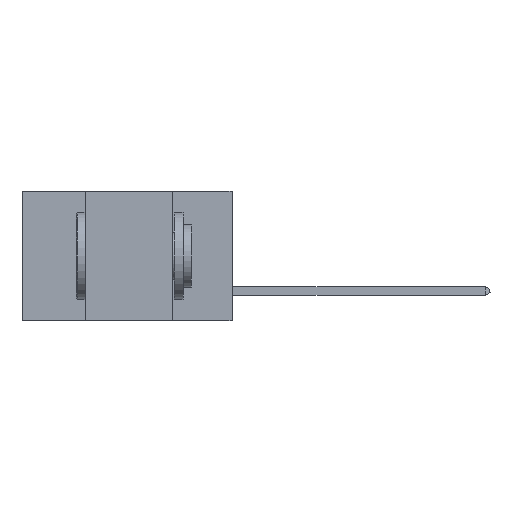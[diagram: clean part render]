
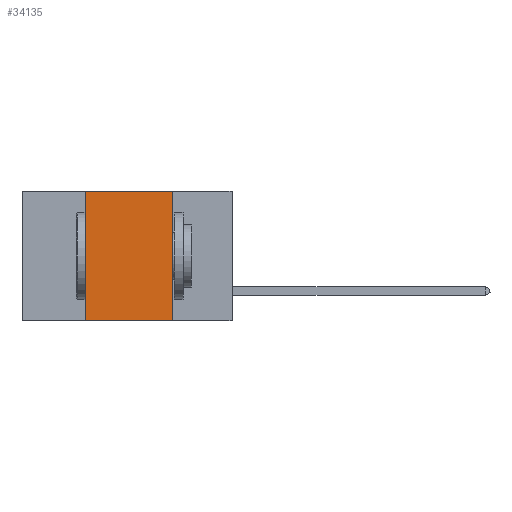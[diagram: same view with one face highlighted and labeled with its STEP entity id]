
A CAD part, left-side view. The second image highlights one B-rep face of the part: STEP entity #34135.
In plain terms, the highlighted planar face has unit normal (-1, 0, 0).
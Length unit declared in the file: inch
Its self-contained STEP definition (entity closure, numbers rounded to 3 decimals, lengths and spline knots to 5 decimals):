
#40 = ORIENTED_EDGE ( 'NONE', *, *, #30660, .F. ) ;
#531 = VERTEX_POINT ( 'NONE', #46135 ) ;
#1060 = DIRECTION ( 'NONE',  ( 0., -1., 0. ) ) ;
#1617 = VERTEX_POINT ( 'NONE', #18326 ) ;
#1627 = VECTOR ( 'NONE', #43679, 39.37008 ) ;
#3214 = CARTESIAN_POINT ( 'NONE',  ( 0., 0.17, 0. ) ) ;
#6801 = DIRECTION ( 'NONE',  ( 1., 0., 0. ) ) ;
#9596 = FACE_OUTER_BOUND ( 'NONE', #28819, .T. ) ;
#10381 = EDGE_CURVE ( 'NONE', #30136, #1617, #22337, .T. ) ;
#11424 = EDGE_CURVE ( 'NONE', #531, #1617, #42454, .T. ) ;
#12493 = VECTOR ( 'NONE', #1060, 39.37008 ) ;
#13430 = DIRECTION ( 'NONE',  ( 0., 0., -1. ) ) ;
#14070 = CARTESIAN_POINT ( 'NONE',  ( 0., 0.17, 0. ) ) ;
#15153 = EDGE_CURVE ( 'NONE', #531, #47347, #36302, .T. ) ;
#15177 = VECTOR ( 'NONE', #28790, 39.37008 ) ;
#17075 = VECTOR ( 'NONE', #13430, 39.37008 ) ;
#17407 = CARTESIAN_POINT ( 'NONE',  ( 0., 0.42, 0. ) ) ;
#18109 = DIRECTION ( 'NONE',  ( 0., 0., -1. ) ) ;
#18326 = CARTESIAN_POINT ( 'NONE',  ( 0., 0.17, -0.37 ) ) ;
#22098 = ORIENTED_EDGE ( 'NONE', *, *, #15153, .F. ) ;
#22337 = LINE ( 'NONE', #14070, #17075 ) ;
#22522 = AXIS2_PLACEMENT_3D ( 'NONE', #29332, #6801, #18109 ) ;
#23462 = CARTESIAN_POINT ( 'NONE',  ( 0., 0.6, -0.37 ) ) ;
#28790 = DIRECTION ( 'NONE',  ( 0., -1., 0. ) ) ;
#28819 = EDGE_LOOP ( 'NONE', ( #30182, #40, #22098, #46249 ) ) ;
#29332 = CARTESIAN_POINT ( 'NONE',  ( 0., 0.6, 0. ) ) ;
#30136 = VERTEX_POINT ( 'NONE', #3214 ) ;
#30182 = ORIENTED_EDGE ( 'NONE', *, *, #10381, .F. ) ;
#30660 = EDGE_CURVE ( 'NONE', #47347, #30136, #45694, .T. ) ;
#34135 = ADVANCED_FACE ( 'NONE', ( #9596 ), #36880, .F. ) ;
#36302 = LINE ( 'NONE', #17407, #1627 ) ;
#36483 = CARTESIAN_POINT ( 'NONE',  ( 0., 0.42, 0. ) ) ;
#36514 = CARTESIAN_POINT ( 'NONE',  ( 0., 0.6, 0. ) ) ;
#36880 = PLANE ( 'NONE',  #22522 ) ;
#42454 = LINE ( 'NONE', #23462, #12493 ) ;
#43679 = DIRECTION ( 'NONE',  ( 0., 0., 1. ) ) ;
#45694 = LINE ( 'NONE', #36514, #15177 ) ;
#46135 = CARTESIAN_POINT ( 'NONE',  ( 0., 0.42, -0.37 ) ) ;
#46249 = ORIENTED_EDGE ( 'NONE', *, *, #11424, .T. ) ;
#47347 = VERTEX_POINT ( 'NONE', #36483 ) ;
